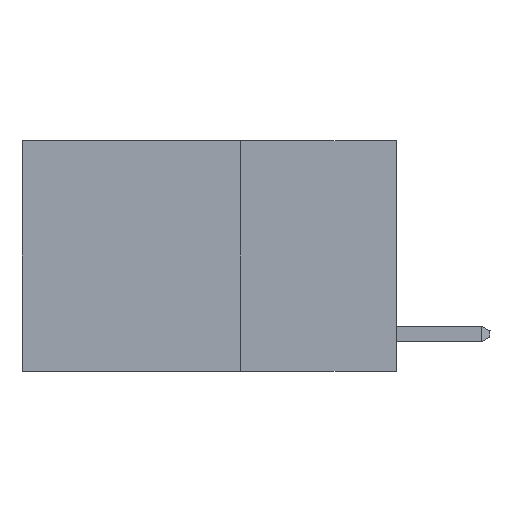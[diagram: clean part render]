
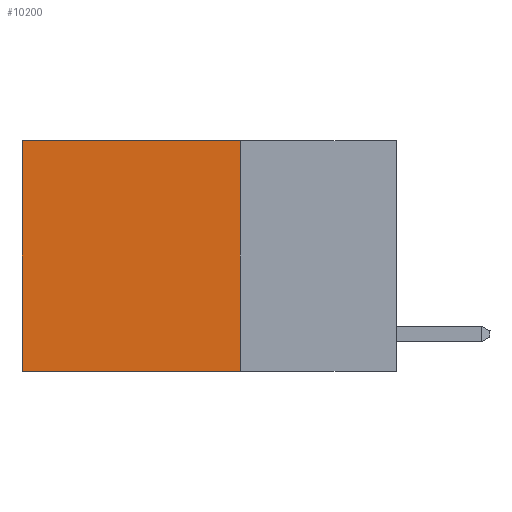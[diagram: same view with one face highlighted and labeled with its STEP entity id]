
A CAD part, left-side view. The second image highlights one B-rep face of the part: STEP entity #10200.
In plain terms, the highlighted planar face has unit normal (-1, 0, 0).
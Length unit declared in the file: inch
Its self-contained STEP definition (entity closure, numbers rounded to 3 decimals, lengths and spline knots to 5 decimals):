
#263 = EDGE_CURVE ( 'NONE', #27350, #10228, #5902, .T. ) ;
#734 = DIRECTION ( 'NONE',  ( 0., 0., -1. ) ) ;
#1539 = LINE ( 'NONE', #24832, #15362 ) ;
#1672 = ORIENTED_EDGE ( 'NONE', *, *, #263, .F. ) ;
#2969 = LINE ( 'NONE', #20652, #22584 ) ;
#3944 = CARTESIAN_POINT ( 'NONE',  ( 0.2625, 0.25, 0. ) ) ;
#5116 = PLANE ( 'NONE',  #6520 ) ;
#5902 = LINE ( 'NONE', #23207, #15551 ) ;
#6520 = AXIS2_PLACEMENT_3D ( 'NONE', #20097, #18025, #27426 ) ;
#6672 = ORIENTED_EDGE ( 'NONE', *, *, #26008, .T. ) ;
#6736 = EDGE_CURVE ( 'NONE', #12113, #27350, #1539, .T. ) ;
#8389 = LINE ( 'NONE', #11563, #17365 ) ;
#10200 = ADVANCED_FACE ( 'NONE', ( #12100 ), #5116, .F. ) ;
#10228 = VERTEX_POINT ( 'NONE', #22791 ) ;
#10645 = ORIENTED_EDGE ( 'NONE', *, *, #17899, .T. ) ;
#11563 = CARTESIAN_POINT ( 'NONE',  ( 0.2625, 0.25, 0. ) ) ;
#11703 = ORIENTED_EDGE ( 'NONE', *, *, #6736, .F. ) ;
#12100 = FACE_OUTER_BOUND ( 'NONE', #18981, .T. ) ;
#12113 = VERTEX_POINT ( 'NONE', #3944 ) ;
#13781 = DIRECTION ( 'NONE',  ( 0., 1., 0. ) ) ;
#14765 = DIRECTION ( 'NONE',  ( 0., 1., 0. ) ) ;
#15260 = VERTEX_POINT ( 'NONE', #18567 ) ;
#15362 = VECTOR ( 'NONE', #26949, 39.37008 ) ;
#15551 = VECTOR ( 'NONE', #14765, 39.37008 ) ;
#17365 = VECTOR ( 'NONE', #13781, 39.37008 ) ;
#17899 = EDGE_CURVE ( 'NONE', #15260, #10228, #2969, .T. ) ;
#18025 = DIRECTION ( 'NONE',  ( 1., 0., 0. ) ) ;
#18567 = CARTESIAN_POINT ( 'NONE',  ( 0.2625, 0.6, 0. ) ) ;
#18981 = EDGE_LOOP ( 'NONE', ( #10645, #1672, #11703, #6672 ) ) ;
#20097 = CARTESIAN_POINT ( 'NONE',  ( 0.2625, 0.25, 0. ) ) ;
#20652 = CARTESIAN_POINT ( 'NONE',  ( 0.2625, 0.6, 0. ) ) ;
#22584 = VECTOR ( 'NONE', #734, 39.37008 ) ;
#22791 = CARTESIAN_POINT ( 'NONE',  ( 0.2625, 0.6, -0.37 ) ) ;
#23207 = CARTESIAN_POINT ( 'NONE',  ( 0.2625, 0.25, -0.37 ) ) ;
#24832 = CARTESIAN_POINT ( 'NONE',  ( 0.2625, 0.25, 0. ) ) ;
#26008 = EDGE_CURVE ( 'NONE', #12113, #15260, #8389, .T. ) ;
#26949 = DIRECTION ( 'NONE',  ( 0., 0., -1. ) ) ;
#27249 = CARTESIAN_POINT ( 'NONE',  ( 0.2625, 0.25, -0.37 ) ) ;
#27350 = VERTEX_POINT ( 'NONE', #27249 ) ;
#27426 = DIRECTION ( 'NONE',  ( 0., 0., -1. ) ) ;
